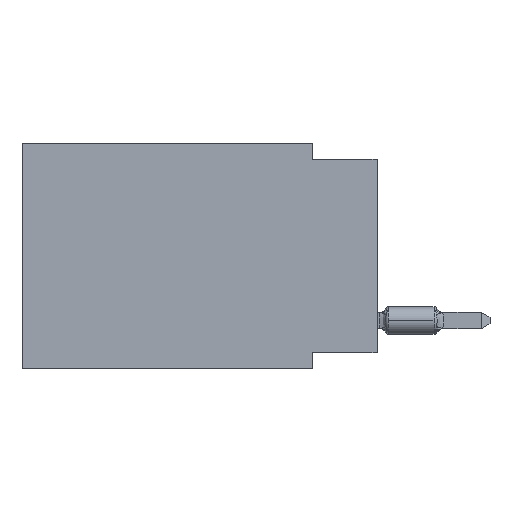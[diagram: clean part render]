
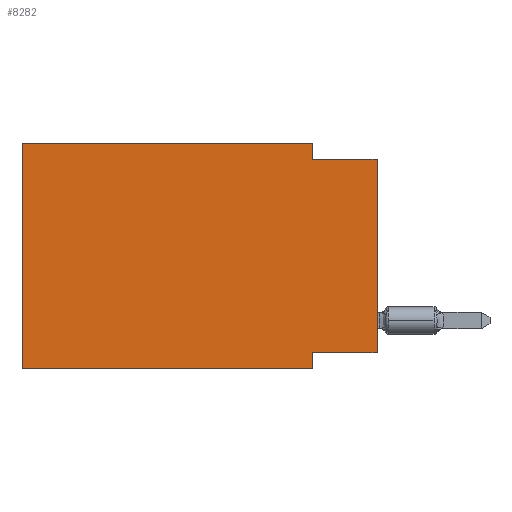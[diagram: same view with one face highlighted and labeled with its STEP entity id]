
A CAD part, left-side view. The second image highlights one B-rep face of the part: STEP entity #8282.
In plain terms, the highlighted planar face has unit normal (-1, 0, 0).
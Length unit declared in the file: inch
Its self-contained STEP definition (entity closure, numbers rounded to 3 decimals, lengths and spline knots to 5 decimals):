
#20 = AXIS2_PLACEMENT_3D ( 'NONE', #1400, #8589, #2456 ) ;
#221 = ORIENTED_EDGE ( 'NONE', *, *, #4829, .F. ) ;
#290 = CARTESIAN_POINT ( 'NONE',  ( 0., 0.1, -0.35 ) ) ;
#497 = VERTEX_POINT ( 'NONE', #8440 ) ;
#558 = CARTESIAN_POINT ( 'NONE',  ( 0., 0.55, -0.35 ) ) ;
#672 = CARTESIAN_POINT ( 'NONE',  ( 0., 0.1, 0. ) ) ;
#1032 = CARTESIAN_POINT ( 'NONE',  ( 0., 0., -0.325 ) ) ;
#1116 = VECTOR ( 'NONE', #10972, 39.37008 ) ;
#1232 = VERTEX_POINT ( 'NONE', #7101 ) ;
#1285 = CARTESIAN_POINT ( 'NONE',  ( 0., 0.55, 0. ) ) ;
#1291 = VECTOR ( 'NONE', #7185, 39.37008 ) ;
#1400 = CARTESIAN_POINT ( 'NONE',  ( 0., 0.55, 0. ) ) ;
#1626 = DIRECTION ( 'NONE',  ( 0., -1., 0. ) ) ;
#1692 = VERTEX_POINT ( 'NONE', #8904 ) ;
#1900 = CARTESIAN_POINT ( 'NONE',  ( 0., 0., 0. ) ) ;
#2050 = DIRECTION ( 'NONE',  ( 0., 0., 1. ) ) ;
#2191 = CARTESIAN_POINT ( 'NONE',  ( 0., 0.55, 0. ) ) ;
#2263 = VECTOR ( 'NONE', #2050, 39.37008 ) ;
#2456 = DIRECTION ( 'NONE',  ( 0., 0., -1. ) ) ;
#2537 = ORIENTED_EDGE ( 'NONE', *, *, #12005, .F. ) ;
#2624 = VERTEX_POINT ( 'NONE', #2191 ) ;
#3112 = EDGE_CURVE ( 'NONE', #497, #1232, #8849, .T. ) ;
#3317 = CARTESIAN_POINT ( 'NONE',  ( 0., 0., -0.025 ) ) ;
#3526 = LINE ( 'NONE', #4987, #8319 ) ;
#3675 = EDGE_CURVE ( 'NONE', #9871, #5624, #9971, .T. ) ;
#4297 = VECTOR ( 'NONE', #10591, 39.37008 ) ;
#4829 = EDGE_CURVE ( 'NONE', #2624, #11415, #10095, .T. ) ;
#4836 = VERTEX_POINT ( 'NONE', #290 ) ;
#4987 = CARTESIAN_POINT ( 'NONE',  ( 0., 0.1, -0.35 ) ) ;
#5082 = CARTESIAN_POINT ( 'NONE',  ( 0., 0.55, 0. ) ) ;
#5606 = ORIENTED_EDGE ( 'NONE', *, *, #10445, .F. ) ;
#5624 = VERTEX_POINT ( 'NONE', #12817 ) ;
#6506 = PLANE ( 'NONE',  #20 ) ;
#7101 = CARTESIAN_POINT ( 'NONE',  ( 0., 0.1, -0.325 ) ) ;
#7185 = DIRECTION ( 'NONE',  ( 0., 1., 0. ) ) ;
#8027 = LINE ( 'NONE', #5082, #2263 ) ;
#8071 = DIRECTION ( 'NONE',  ( 0., 0., -1. ) ) ;
#8076 = DIRECTION ( 'NONE',  ( 0., 0., 1. ) ) ;
#8282 = ADVANCED_FACE ( 'NONE', ( #13274 ), #6506, .F. ) ;
#8319 = VECTOR ( 'NONE', #8071, 39.37008 ) ;
#8393 = ORIENTED_EDGE ( 'NONE', *, *, #11150, .T. ) ;
#8440 = CARTESIAN_POINT ( 'NONE',  ( 0., 0., -0.325 ) ) ;
#8508 = ORIENTED_EDGE ( 'NONE', *, *, #11638, .T. ) ;
#8589 = DIRECTION ( 'NONE',  ( 1., 0., 0. ) ) ;
#8849 = LINE ( 'NONE', #1032, #1291 ) ;
#8904 = CARTESIAN_POINT ( 'NONE',  ( 0., 0.55, -0.35 ) ) ;
#9131 = EDGE_LOOP ( 'NONE', ( #8393, #11386, #11544, #221, #5606, #8508, #2537, #10969 ) ) ;
#9519 = DIRECTION ( 'NONE',  ( 0., -1., 0. ) ) ;
#9871 = VERTEX_POINT ( 'NONE', #11306 ) ;
#9971 = LINE ( 'NONE', #3317, #12359 ) ;
#10095 = LINE ( 'NONE', #1285, #4297 ) ;
#10127 = VECTOR ( 'NONE', #1626, 39.37008 ) ;
#10445 = EDGE_CURVE ( 'NONE', #1692, #2624, #8027, .T. ) ;
#10456 = VECTOR ( 'NONE', #8076, 39.37008 ) ;
#10591 = DIRECTION ( 'NONE',  ( 0., -1., 0. ) ) ;
#10969 = ORIENTED_EDGE ( 'NONE', *, *, #3112, .F. ) ;
#10972 = DIRECTION ( 'NONE',  ( 0., 0., -1. ) ) ;
#11024 = EDGE_CURVE ( 'NONE', #11415, #9871, #12063, .T. ) ;
#11150 = EDGE_CURVE ( 'NONE', #497, #5624, #12856, .T. ) ;
#11306 = CARTESIAN_POINT ( 'NONE',  ( 0., 0.1, -0.025 ) ) ;
#11386 = ORIENTED_EDGE ( 'NONE', *, *, #3675, .F. ) ;
#11415 = VERTEX_POINT ( 'NONE', #12562 ) ;
#11544 = ORIENTED_EDGE ( 'NONE', *, *, #11024, .F. ) ;
#11638 = EDGE_CURVE ( 'NONE', #1692, #4836, #12840, .T. ) ;
#12005 = EDGE_CURVE ( 'NONE', #1232, #4836, #3526, .T. ) ;
#12063 = LINE ( 'NONE', #672, #1116 ) ;
#12359 = VECTOR ( 'NONE', #9519, 39.37008 ) ;
#12562 = CARTESIAN_POINT ( 'NONE',  ( 0., 0.1, 0. ) ) ;
#12817 = CARTESIAN_POINT ( 'NONE',  ( 0., 0., -0.025 ) ) ;
#12840 = LINE ( 'NONE', #558, #10127 ) ;
#12856 = LINE ( 'NONE', #1900, #10456 ) ;
#13274 = FACE_OUTER_BOUND ( 'NONE', #9131, .T. ) ;
